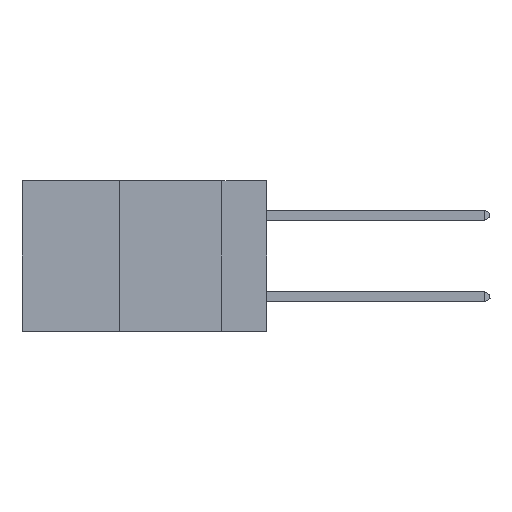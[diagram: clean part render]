
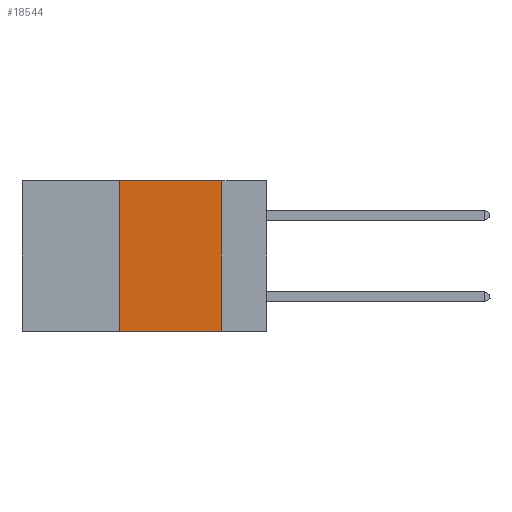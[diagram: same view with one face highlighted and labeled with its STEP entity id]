
A CAD part, left-side view. The second image highlights one B-rep face of the part: STEP entity #18544.
In plain terms, the highlighted planar face has unit normal (-1, 0, 0).
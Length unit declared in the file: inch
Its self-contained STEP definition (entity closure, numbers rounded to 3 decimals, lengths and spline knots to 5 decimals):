
#2379 = VECTOR ( 'NONE', #26236, 39.37008 ) ;
#2767 = VECTOR ( 'NONE', #31532, 39.37008 ) ;
#3505 = VERTEX_POINT ( 'NONE', #23533 ) ;
#8129 = CARTESIAN_POINT ( 'NONE',  ( 0., 0.6, 0. ) ) ;
#8370 = DIRECTION ( 'NONE',  ( 0., 0., -1. ) ) ;
#10125 = ORIENTED_EDGE ( 'NONE', *, *, #19784, .F. ) ;
#10905 = CARTESIAN_POINT ( 'NONE',  ( 0., 0.11, -0.37 ) ) ;
#10919 = VERTEX_POINT ( 'NONE', #10905 ) ;
#11778 = ORIENTED_EDGE ( 'NONE', *, *, #15149, .T. ) ;
#13622 = LINE ( 'NONE', #27963, #2767 ) ;
#14353 = ORIENTED_EDGE ( 'NONE', *, *, #15223, .F. ) ;
#15149 = EDGE_CURVE ( 'NONE', #30660, #10919, #13622, .T. ) ;
#15223 = EDGE_CURVE ( 'NONE', #30660, #3505, #36602, .T. ) ;
#15279 = EDGE_CURVE ( 'NONE', #33013, #10919, #17618, .T. ) ;
#15336 = VECTOR ( 'NONE', #21576, 39.37008 ) ;
#15964 = EDGE_LOOP ( 'NONE', ( #35230, #10125, #14353, #11778 ) ) ;
#17618 = LINE ( 'NONE', #25171, #15336 ) ;
#18544 = ADVANCED_FACE ( 'NONE', ( #22903 ), #29895, .F. ) ;
#19784 = EDGE_CURVE ( 'NONE', #3505, #33013, #40694, .T. ) ;
#21576 = DIRECTION ( 'NONE',  ( 0., 0., -1. ) ) ;
#22903 = FACE_OUTER_BOUND ( 'NONE', #15964, .T. ) ;
#23533 = CARTESIAN_POINT ( 'NONE',  ( 0., 0.36, 0. ) ) ;
#25171 = CARTESIAN_POINT ( 'NONE',  ( 0., 0.11, 0. ) ) ;
#26236 = DIRECTION ( 'NONE',  ( 0., -1., 0. ) ) ;
#26483 = CARTESIAN_POINT ( 'NONE',  ( 0., 0.6, 0. ) ) ;
#27120 = VECTOR ( 'NONE', #42650, 39.37008 ) ;
#27788 = CARTESIAN_POINT ( 'NONE',  ( 0., 0.36, -0.37 ) ) ;
#27963 = CARTESIAN_POINT ( 'NONE',  ( 0., 0.6, -0.37 ) ) ;
#29895 = PLANE ( 'NONE',  #30561 ) ;
#30047 = DIRECTION ( 'NONE',  ( 1., 0., 0. ) ) ;
#30561 = AXIS2_PLACEMENT_3D ( 'NONE', #26483, #30047, #8370 ) ;
#30660 = VERTEX_POINT ( 'NONE', #27788 ) ;
#31532 = DIRECTION ( 'NONE',  ( 0., -1., 0. ) ) ;
#33013 = VERTEX_POINT ( 'NONE', #33203 ) ;
#33203 = CARTESIAN_POINT ( 'NONE',  ( 0., 0.11, 0. ) ) ;
#35230 = ORIENTED_EDGE ( 'NONE', *, *, #15279, .F. ) ;
#36602 = LINE ( 'NONE', #39018, #27120 ) ;
#39018 = CARTESIAN_POINT ( 'NONE',  ( 0., 0.36, 0. ) ) ;
#40694 = LINE ( 'NONE', #8129, #2379 ) ;
#42650 = DIRECTION ( 'NONE',  ( 0., 0., 1. ) ) ;
